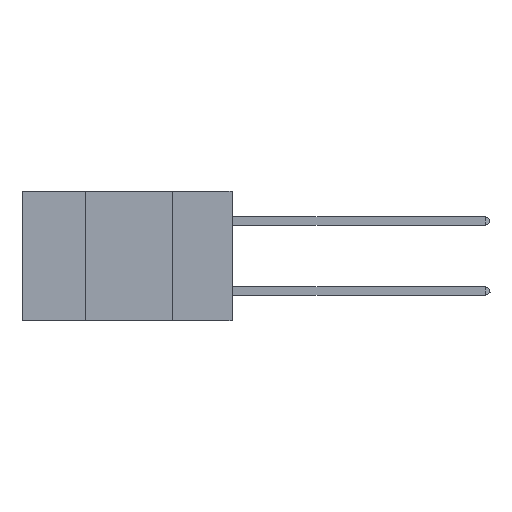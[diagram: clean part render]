
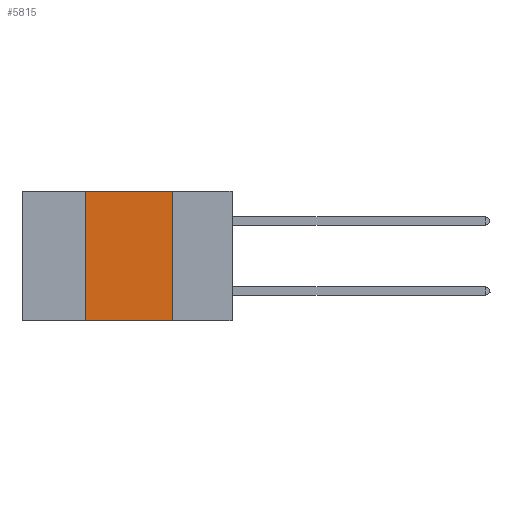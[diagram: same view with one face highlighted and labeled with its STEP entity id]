
A CAD part, left-side view. The second image highlights one B-rep face of the part: STEP entity #5815.
In plain terms, the highlighted planar face has unit normal (-1, 0, 0).
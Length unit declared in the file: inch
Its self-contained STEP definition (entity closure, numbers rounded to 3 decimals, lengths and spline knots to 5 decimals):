
#336 = CARTESIAN_POINT ( 'NONE',  ( 0., 0.17, 0. ) ) ;
#2247 = ORIENTED_EDGE ( 'NONE', *, *, #4561, .F. ) ;
#2369 = VERTEX_POINT ( 'NONE', #336 ) ;
#2389 = DIRECTION ( 'NONE',  ( 0., 0., -1. ) ) ;
#3430 = LINE ( 'NONE', #7121, #17364 ) ;
#3640 = VECTOR ( 'NONE', #11407, 39.37008 ) ;
#4129 = AXIS2_PLACEMENT_3D ( 'NONE', #9262, #6416, #2389 ) ;
#4203 = CARTESIAN_POINT ( 'NONE',  ( 0., 0.42, 0. ) ) ;
#4561 = EDGE_CURVE ( 'NONE', #2369, #8198, #8687, .T. ) ;
#5815 = ADVANCED_FACE ( 'NONE', ( #13867 ), #14552, .F. ) ;
#6278 = VERTEX_POINT ( 'NONE', #9325 ) ;
#6416 = DIRECTION ( 'NONE',  ( 1., 0., 0. ) ) ;
#7121 = CARTESIAN_POINT ( 'NONE',  ( 0., 0.6, 0. ) ) ;
#7254 = LINE ( 'NONE', #11327, #3640 ) ;
#7628 = VERTEX_POINT ( 'NONE', #11431 ) ;
#8198 = VERTEX_POINT ( 'NONE', #8848 ) ;
#8462 = LINE ( 'NONE', #4203, #14592 ) ;
#8687 = LINE ( 'NONE', #14998, #9741 ) ;
#8848 = CARTESIAN_POINT ( 'NONE',  ( 0., 0.17, -0.37 ) ) ;
#9154 = EDGE_CURVE ( 'NONE', #6278, #2369, #3430, .T. ) ;
#9262 = CARTESIAN_POINT ( 'NONE',  ( 0., 0.6, 0. ) ) ;
#9325 = CARTESIAN_POINT ( 'NONE',  ( 0., 0.42, 0. ) ) ;
#9741 = VECTOR ( 'NONE', #13398, 39.37008 ) ;
#11327 = CARTESIAN_POINT ( 'NONE',  ( 0., 0.6, -0.37 ) ) ;
#11407 = DIRECTION ( 'NONE',  ( 0., -1., 0. ) ) ;
#11431 = CARTESIAN_POINT ( 'NONE',  ( 0., 0.42, -0.37 ) ) ;
#12197 = EDGE_LOOP ( 'NONE', ( #2247, #17466, #12944, #17441 ) ) ;
#12944 = ORIENTED_EDGE ( 'NONE', *, *, #14030, .F. ) ;
#13129 = EDGE_CURVE ( 'NONE', #7628, #8198, #7254, .T. ) ;
#13398 = DIRECTION ( 'NONE',  ( 0., 0., -1. ) ) ;
#13867 = FACE_OUTER_BOUND ( 'NONE', #12197, .T. ) ;
#14030 = EDGE_CURVE ( 'NONE', #7628, #6278, #8462, .T. ) ;
#14412 = DIRECTION ( 'NONE',  ( 0., 0., 1. ) ) ;
#14552 = PLANE ( 'NONE',  #4129 ) ;
#14592 = VECTOR ( 'NONE', #14412, 39.37008 ) ;
#14998 = CARTESIAN_POINT ( 'NONE',  ( 0., 0.17, 0. ) ) ;
#15305 = DIRECTION ( 'NONE',  ( 0., -1., 0. ) ) ;
#17364 = VECTOR ( 'NONE', #15305, 39.37008 ) ;
#17441 = ORIENTED_EDGE ( 'NONE', *, *, #13129, .T. ) ;
#17466 = ORIENTED_EDGE ( 'NONE', *, *, #9154, .F. ) ;
